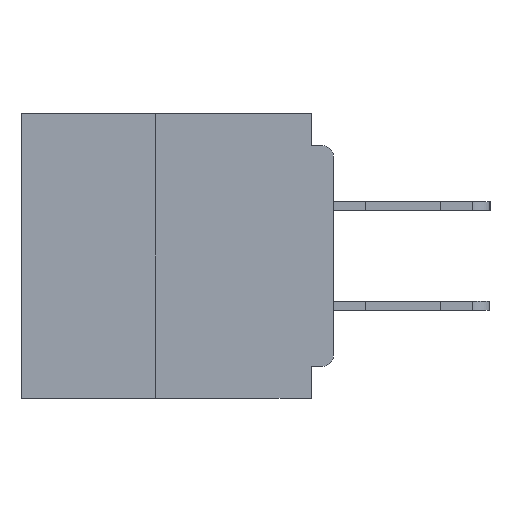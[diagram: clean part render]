
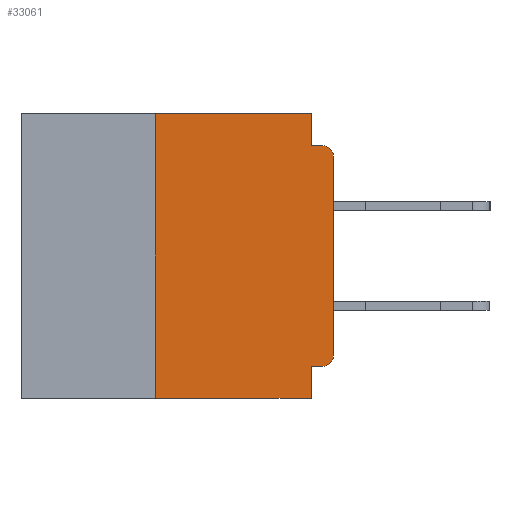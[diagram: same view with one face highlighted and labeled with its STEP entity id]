
A CAD part, left-side view. The second image highlights one B-rep face of the part: STEP entity #33061.
In plain terms, the highlighted planar face has unit normal (-1, 0, 0).
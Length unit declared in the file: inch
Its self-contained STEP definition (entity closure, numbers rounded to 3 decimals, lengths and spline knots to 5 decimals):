
#437 = CARTESIAN_POINT ( 'NONE',  ( 0., 0.015, -0.355 ) ) ;
#892 = VECTOR ( 'NONE', #32132, 39.37008 ) ;
#1397 = VECTOR ( 'NONE', #18558, 39.37008 ) ;
#1527 = DIRECTION ( 'NONE',  ( 0., -1., 0. ) ) ;
#1927 = DIRECTION ( 'NONE',  ( 0., 0., -1. ) ) ;
#3096 = CARTESIAN_POINT ( 'NONE',  ( 0., 0.015, -0.34 ) ) ;
#5148 = VECTOR ( 'NONE', #30694, 39.37008 ) ;
#5404 = CARTESIAN_POINT ( 'NONE',  ( 0., 0.031, -0.355 ) ) ;
#5596 = ORIENTED_EDGE ( 'NONE', *, *, #38308, .F. ) ;
#6362 = DIRECTION ( 'NONE',  ( 0., 0., -1. ) ) ;
#6926 = VERTEX_POINT ( 'NONE', #14049 ) ;
#7336 = AXIS2_PLACEMENT_3D ( 'NONE', #10012, #32530, #13217 ) ;
#7476 = CARTESIAN_POINT ( 'NONE',  ( 0., 0.25, -0.4 ) ) ;
#7932 = EDGE_CURVE ( 'NONE', #38635, #15261, #10959, .T. ) ;
#8454 = DIRECTION ( 'NONE',  ( 0., 1., 0. ) ) ;
#9441 = LINE ( 'NONE', #35182, #892 ) ;
#9901 = EDGE_CURVE ( 'NONE', #15138, #16171, #18779, .T. ) ;
#10012 = CARTESIAN_POINT ( 'NONE',  ( 0., 0.015, -0.06 ) ) ;
#10959 = LINE ( 'NONE', #28177, #1397 ) ;
#11165 = LINE ( 'NONE', #23759, #15566 ) ;
#11629 = ORIENTED_EDGE ( 'NONE', *, *, #9901, .T. ) ;
#11731 = CARTESIAN_POINT ( 'NONE',  ( 0., 0.25, -0.4 ) ) ;
#12109 = ORIENTED_EDGE ( 'NONE', *, *, #7932, .F. ) ;
#13142 = CARTESIAN_POINT ( 'NONE',  ( 0., 0.031, -0.045 ) ) ;
#13217 = DIRECTION ( 'NONE',  ( 0., 0., -1. ) ) ;
#13807 = AXIS2_PLACEMENT_3D ( 'NONE', #17931, #21174, #1927 ) ;
#14012 = CARTESIAN_POINT ( 'NONE',  ( 0., 0.437, 0. ) ) ;
#14049 = CARTESIAN_POINT ( 'NONE',  ( 0., 0.031, -0.4 ) ) ;
#14119 = ORIENTED_EDGE ( 'NONE', *, *, #26527, .F. ) ;
#14172 = DIRECTION ( 'NONE',  ( 0., 0., -1. ) ) ;
#14275 = CARTESIAN_POINT ( 'NONE',  ( 0., 0.437, -0.4 ) ) ;
#15138 = VERTEX_POINT ( 'NONE', #437 ) ;
#15261 = VERTEX_POINT ( 'NONE', #33236 ) ;
#15425 = VERTEX_POINT ( 'NONE', #24479 ) ;
#15566 = VECTOR ( 'NONE', #14172, 39.37008 ) ;
#15680 = LINE ( 'NONE', #24063, #5148 ) ;
#16134 = LINE ( 'NONE', #14275, #32284 ) ;
#16171 = VERTEX_POINT ( 'NONE', #24715 ) ;
#17931 = CARTESIAN_POINT ( 'NONE',  ( 0., 0.437, 0. ) ) ;
#18558 = DIRECTION ( 'NONE',  ( 0., -1., 0. ) ) ;
#18779 = CIRCLE ( 'NONE', #31047, 0.015 ) ;
#19005 = EDGE_LOOP ( 'NONE', ( #39222, #23182, #12109, #20662, #5596, #14119, #22681, #33297, #36272, #11629 ) ) ;
#19034 = EDGE_CURVE ( 'NONE', #15425, #15261, #24362, .T. ) ;
#20662 = ORIENTED_EDGE ( 'NONE', *, *, #24348, .F. ) ;
#21174 = DIRECTION ( 'NONE',  ( 1., 0., 0. ) ) ;
#22681 = ORIENTED_EDGE ( 'NONE', *, *, #32988, .T. ) ;
#23182 = ORIENTED_EDGE ( 'NONE', *, *, #19034, .T. ) ;
#23759 = CARTESIAN_POINT ( 'NONE',  ( 0., 0.031, 0. ) ) ;
#24063 = CARTESIAN_POINT ( 'NONE',  ( 0., 0., 0. ) ) ;
#24133 = VECTOR ( 'NONE', #39704, 39.37008 ) ;
#24348 = EDGE_CURVE ( 'NONE', #36973, #38635, #11165, .T. ) ;
#24362 = CIRCLE ( 'NONE', #7336, 0.015 ) ;
#24479 = CARTESIAN_POINT ( 'NONE',  ( 0., 0., -0.06 ) ) ;
#24536 = LINE ( 'NONE', #11731, #40516 ) ;
#24694 = DIRECTION ( 'NONE',  ( 0., 0., 1. ) ) ;
#24715 = CARTESIAN_POINT ( 'NONE',  ( 0., 0., -0.34 ) ) ;
#25153 = LINE ( 'NONE', #14012, #24133 ) ;
#25637 = DIRECTION ( 'NONE',  ( -1., 0., 0. ) ) ;
#26527 = EDGE_CURVE ( 'NONE', #30547, #26636, #24536, .T. ) ;
#26636 = VERTEX_POINT ( 'NONE', #34910 ) ;
#28177 = CARTESIAN_POINT ( 'NONE',  ( 0., 0., -0.045 ) ) ;
#28759 = LINE ( 'NONE', #34174, #37234 ) ;
#30061 = CARTESIAN_POINT ( 'NONE',  ( 0., 0.031, 0. ) ) ;
#30142 = EDGE_CURVE ( 'NONE', #15138, #39034, #28759, .T. ) ;
#30547 = VERTEX_POINT ( 'NONE', #7476 ) ;
#30694 = DIRECTION ( 'NONE',  ( 0., 0., 1. ) ) ;
#31047 = AXIS2_PLACEMENT_3D ( 'NONE', #3096, #25637, #6362 ) ;
#31282 = FACE_OUTER_BOUND ( 'NONE', #19005, .T. ) ;
#32132 = DIRECTION ( 'NONE',  ( 0., 0., -1. ) ) ;
#32284 = VECTOR ( 'NONE', #1527, 39.37008 ) ;
#32416 = EDGE_CURVE ( 'NONE', #16171, #15425, #15680, .T. ) ;
#32530 = DIRECTION ( 'NONE',  ( -1., 0., 0. ) ) ;
#32988 = EDGE_CURVE ( 'NONE', #30547, #6926, #16134, .T. ) ;
#33061 = ADVANCED_FACE ( 'NONE', ( #31282 ), #37172, .F. ) ;
#33236 = CARTESIAN_POINT ( 'NONE',  ( 0., 0.015, -0.045 ) ) ;
#33297 = ORIENTED_EDGE ( 'NONE', *, *, #35090, .F. ) ;
#34174 = CARTESIAN_POINT ( 'NONE',  ( 0., 0., -0.355 ) ) ;
#34910 = CARTESIAN_POINT ( 'NONE',  ( 0., 0.25, 0. ) ) ;
#35090 = EDGE_CURVE ( 'NONE', #39034, #6926, #9441, .T. ) ;
#35182 = CARTESIAN_POINT ( 'NONE',  ( 0., 0.031, -0.4 ) ) ;
#36272 = ORIENTED_EDGE ( 'NONE', *, *, #30142, .F. ) ;
#36973 = VERTEX_POINT ( 'NONE', #30061 ) ;
#37172 = PLANE ( 'NONE',  #13807 ) ;
#37234 = VECTOR ( 'NONE', #8454, 39.37008 ) ;
#38308 = EDGE_CURVE ( 'NONE', #26636, #36973, #25153, .T. ) ;
#38635 = VERTEX_POINT ( 'NONE', #13142 ) ;
#39034 = VERTEX_POINT ( 'NONE', #5404 ) ;
#39222 = ORIENTED_EDGE ( 'NONE', *, *, #32416, .T. ) ;
#39704 = DIRECTION ( 'NONE',  ( 0., -1., 0. ) ) ;
#40516 = VECTOR ( 'NONE', #24694, 39.37008 ) ;
